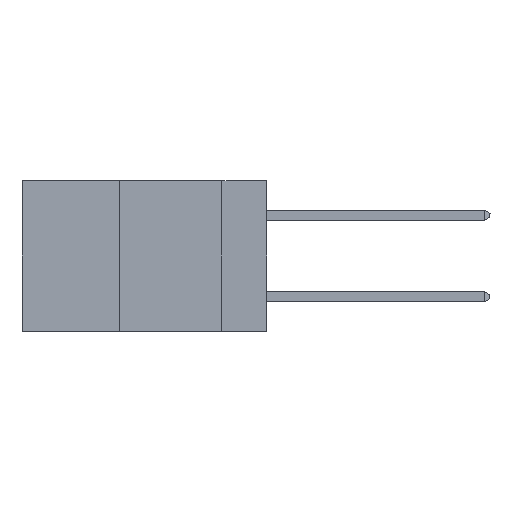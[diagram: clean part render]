
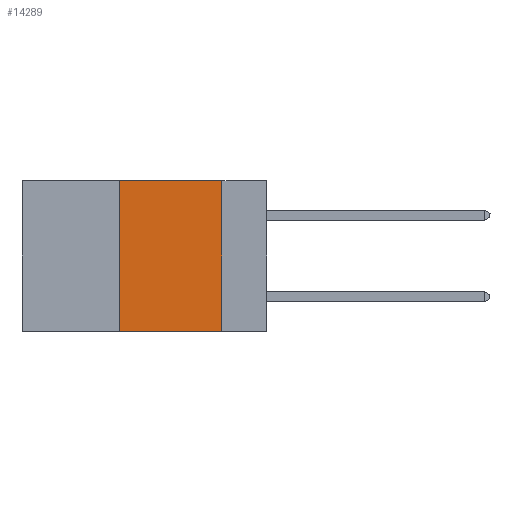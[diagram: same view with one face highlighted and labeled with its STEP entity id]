
A CAD part, left-side view. The second image highlights one B-rep face of the part: STEP entity #14289.
In plain terms, the highlighted planar face has unit normal (-1, 0, 0).
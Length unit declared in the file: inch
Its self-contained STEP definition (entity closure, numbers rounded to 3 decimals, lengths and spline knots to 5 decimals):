
#501 = DIRECTION ( 'NONE',  ( 0., 0., 1. ) ) ;
#1134 = VECTOR ( 'NONE', #18305, 39.37008 ) ;
#1928 = LINE ( 'NONE', #17167, #17313 ) ;
#2088 = EDGE_CURVE ( 'NONE', #9565, #24713, #16313, .T. ) ;
#2566 = VECTOR ( 'NONE', #14005, 39.37008 ) ;
#3312 = ORIENTED_EDGE ( 'NONE', *, *, #2088, .F. ) ;
#5079 = VECTOR ( 'NONE', #501, 39.37008 ) ;
#5941 = CARTESIAN_POINT ( 'NONE',  ( 0., 0.11, 0. ) ) ;
#7990 = LINE ( 'NONE', #5941, #2566 ) ;
#8039 = ORIENTED_EDGE ( 'NONE', *, *, #20024, .T. ) ;
#8861 = ORIENTED_EDGE ( 'NONE', *, *, #10575, .F. ) ;
#9565 = VERTEX_POINT ( 'NONE', #24322 ) ;
#9724 = PLANE ( 'NONE',  #18044 ) ;
#10509 = VERTEX_POINT ( 'NONE', #25239 ) ;
#10575 = EDGE_CURVE ( 'NONE', #25432, #10509, #7990, .T. ) ;
#13123 = FACE_OUTER_BOUND ( 'NONE', #15772, .T. ) ;
#13582 = CARTESIAN_POINT ( 'NONE',  ( 0., 0.11, 0. ) ) ;
#13745 = DIRECTION ( 'NONE',  ( 0., 0., -1. ) ) ;
#14005 = DIRECTION ( 'NONE',  ( 0., 0., -1. ) ) ;
#14289 = ADVANCED_FACE ( 'NONE', ( #13123 ), #9724, .F. ) ;
#15431 = CARTESIAN_POINT ( 'NONE',  ( 0., 0.36, 0. ) ) ;
#15646 = CARTESIAN_POINT ( 'NONE',  ( 0., 0.6, 0. ) ) ;
#15772 = EDGE_LOOP ( 'NONE', ( #8861, #19001, #3312, #8039 ) ) ;
#16313 = LINE ( 'NONE', #21584, #5079 ) ;
#17167 = CARTESIAN_POINT ( 'NONE',  ( 0., 0.6, 0. ) ) ;
#17313 = VECTOR ( 'NONE', #19150, 39.37008 ) ;
#18044 = AXIS2_PLACEMENT_3D ( 'NONE', #15646, #21493, #13745 ) ;
#18305 = DIRECTION ( 'NONE',  ( 0., -1., 0. ) ) ;
#19001 = ORIENTED_EDGE ( 'NONE', *, *, #23980, .F. ) ;
#19150 = DIRECTION ( 'NONE',  ( 0., -1., 0. ) ) ;
#20024 = EDGE_CURVE ( 'NONE', #9565, #10509, #22996, .T. ) ;
#21493 = DIRECTION ( 'NONE',  ( 1., 0., 0. ) ) ;
#21584 = CARTESIAN_POINT ( 'NONE',  ( 0., 0.36, 0. ) ) ;
#22249 = CARTESIAN_POINT ( 'NONE',  ( 0., 0.6, -0.37 ) ) ;
#22996 = LINE ( 'NONE', #22249, #1134 ) ;
#23980 = EDGE_CURVE ( 'NONE', #24713, #25432, #1928, .T. ) ;
#24322 = CARTESIAN_POINT ( 'NONE',  ( 0., 0.36, -0.37 ) ) ;
#24713 = VERTEX_POINT ( 'NONE', #15431 ) ;
#25239 = CARTESIAN_POINT ( 'NONE',  ( 0., 0.11, -0.37 ) ) ;
#25432 = VERTEX_POINT ( 'NONE', #13582 ) ;
